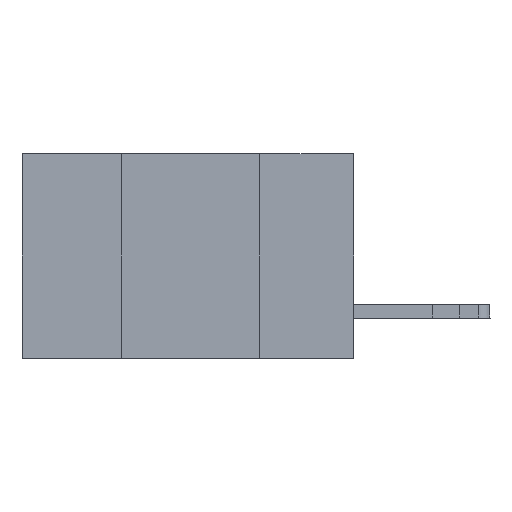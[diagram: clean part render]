
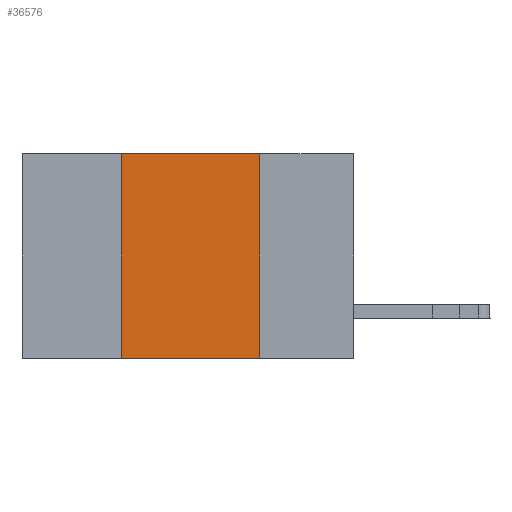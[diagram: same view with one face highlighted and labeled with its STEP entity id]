
A CAD part, left-side view. The second image highlights one B-rep face of the part: STEP entity #36576.
In plain terms, the highlighted planar face has unit normal (-1, 0, 0).
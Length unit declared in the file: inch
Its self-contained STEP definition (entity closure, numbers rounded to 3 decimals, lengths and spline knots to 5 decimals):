
#2612 = CARTESIAN_POINT ( 'NONE',  ( 0., 0.42, 0. ) ) ;
#2787 = ORIENTED_EDGE ( 'NONE', *, *, #22672, .F. ) ;
#4580 = CARTESIAN_POINT ( 'NONE',  ( 0., 0.42, -0.37 ) ) ;
#4705 = LINE ( 'NONE', #8372, #11690 ) ;
#4863 = EDGE_CURVE ( 'NONE', #23708, #12911, #15887, .T. ) ;
#6482 = LINE ( 'NONE', #25833, #29690 ) ;
#7443 = LINE ( 'NONE', #19186, #19041 ) ;
#8328 = DIRECTION ( 'NONE',  ( 0., -1., 0. ) ) ;
#8372 = CARTESIAN_POINT ( 'NONE',  ( 0., 0.17, 0. ) ) ;
#11613 = DIRECTION ( 'NONE',  ( 0., 0., -1. ) ) ;
#11690 = VECTOR ( 'NONE', #17769, 39.37008 ) ;
#11747 = DIRECTION ( 'NONE',  ( 1., 0., 0. ) ) ;
#12307 = EDGE_CURVE ( 'NONE', #12911, #32274, #7443, .T. ) ;
#12534 = EDGE_CURVE ( 'NONE', #23708, #32029, #6482, .T. ) ;
#12911 = VERTEX_POINT ( 'NONE', #24025 ) ;
#15092 = FACE_OUTER_BOUND ( 'NONE', #36505, .T. ) ;
#15762 = ORIENTED_EDGE ( 'NONE', *, *, #12307, .F. ) ;
#15887 = LINE ( 'NONE', #2612, #16379 ) ;
#16379 = VECTOR ( 'NONE', #20620, 39.37008 ) ;
#17769 = DIRECTION ( 'NONE',  ( 0., 0., -1. ) ) ;
#19041 = VECTOR ( 'NONE', #28128, 39.37008 ) ;
#19186 = CARTESIAN_POINT ( 'NONE',  ( 0., 0.6, 0. ) ) ;
#20620 = DIRECTION ( 'NONE',  ( 0., 0., 1. ) ) ;
#22672 = EDGE_CURVE ( 'NONE', #32274, #32029, #4705, .T. ) ;
#23659 = PLANE ( 'NONE',  #34085 ) ;
#23708 = VERTEX_POINT ( 'NONE', #4580 ) ;
#24025 = CARTESIAN_POINT ( 'NONE',  ( 0., 0.42, 0. ) ) ;
#25436 = CARTESIAN_POINT ( 'NONE',  ( 0., 0.17, 0. ) ) ;
#25833 = CARTESIAN_POINT ( 'NONE',  ( 0., 0.6, -0.37 ) ) ;
#28128 = DIRECTION ( 'NONE',  ( 0., -1., 0. ) ) ;
#29690 = VECTOR ( 'NONE', #8328, 39.37008 ) ;
#32029 = VERTEX_POINT ( 'NONE', #35757 ) ;
#32274 = VERTEX_POINT ( 'NONE', #25436 ) ;
#32461 = ORIENTED_EDGE ( 'NONE', *, *, #4863, .F. ) ;
#34085 = AXIS2_PLACEMENT_3D ( 'NONE', #38085, #11747, #11613 ) ;
#34762 = ORIENTED_EDGE ( 'NONE', *, *, #12534, .T. ) ;
#35757 = CARTESIAN_POINT ( 'NONE',  ( 0., 0.17, -0.37 ) ) ;
#36505 = EDGE_LOOP ( 'NONE', ( #2787, #15762, #32461, #34762 ) ) ;
#36576 = ADVANCED_FACE ( 'NONE', ( #15092 ), #23659, .F. ) ;
#38085 = CARTESIAN_POINT ( 'NONE',  ( 0., 0.6, 0. ) ) ;
